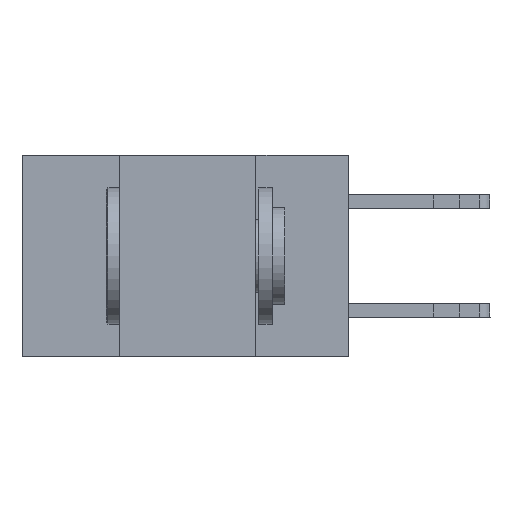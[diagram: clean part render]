
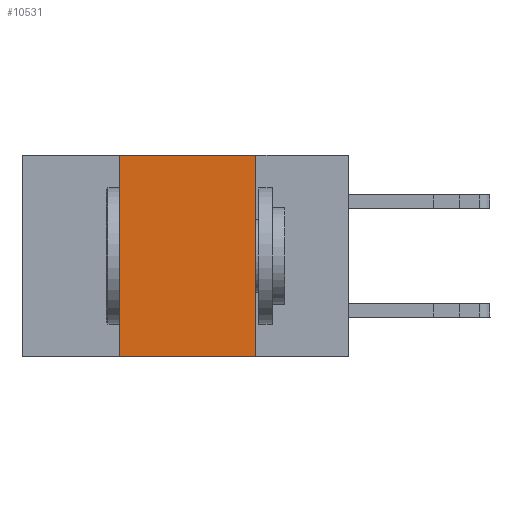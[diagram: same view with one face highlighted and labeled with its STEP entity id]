
A CAD part, left-side view. The second image highlights one B-rep face of the part: STEP entity #10531.
In plain terms, the highlighted planar face has unit normal (-1, 0, 0).
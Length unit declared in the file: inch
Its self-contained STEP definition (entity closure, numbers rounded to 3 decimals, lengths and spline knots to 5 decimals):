
#219 = DIRECTION ( 'NONE',  ( 0., 0., 1. ) ) ;
#605 = CARTESIAN_POINT ( 'NONE',  ( 0., 0.42, 0. ) ) ;
#889 = LINE ( 'NONE', #16623, #11078 ) ;
#1057 = DIRECTION ( 'NONE',  ( 1., 0., 0. ) ) ;
#1347 = DIRECTION ( 'NONE',  ( 0., 0., -1. ) ) ;
#1419 = EDGE_CURVE ( 'NONE', #9690, #16868, #15950, .T. ) ;
#1457 = CARTESIAN_POINT ( 'NONE',  ( 0., 0.6, 0. ) ) ;
#2435 = ORIENTED_EDGE ( 'NONE', *, *, #16948, .F. ) ;
#3744 = VECTOR ( 'NONE', #219, 39.37008 ) ;
#3847 = ORIENTED_EDGE ( 'NONE', *, *, #14532, .F. ) ;
#4110 = ORIENTED_EDGE ( 'NONE', *, *, #1419, .F. ) ;
#4305 = VECTOR ( 'NONE', #15871, 39.37008 ) ;
#4317 = PLANE ( 'NONE',  #13071 ) ;
#4586 = VECTOR ( 'NONE', #1347, 39.37008 ) ;
#4807 = CARTESIAN_POINT ( 'NONE',  ( 0., 0.6, 0. ) ) ;
#5170 = CARTESIAN_POINT ( 'NONE',  ( 0., 0.17, -0.37 ) ) ;
#5462 = EDGE_CURVE ( 'NONE', #10957, #16868, #889, .T. ) ;
#5676 = ORIENTED_EDGE ( 'NONE', *, *, #5462, .T. ) ;
#6406 = FACE_OUTER_BOUND ( 'NONE', #16677, .T. ) ;
#7031 = CARTESIAN_POINT ( 'NONE',  ( 0., 0.42, -0.37 ) ) ;
#7181 = LINE ( 'NONE', #1457, #4305 ) ;
#7282 = LINE ( 'NONE', #13332, #3744 ) ;
#7953 = CARTESIAN_POINT ( 'NONE',  ( 0., 0.17, 0. ) ) ;
#8764 = VERTEX_POINT ( 'NONE', #605 ) ;
#9690 = VERTEX_POINT ( 'NONE', #11444 ) ;
#10531 = ADVANCED_FACE ( 'NONE', ( #6406 ), #4317, .F. ) ;
#10957 = VERTEX_POINT ( 'NONE', #7031 ) ;
#11078 = VECTOR ( 'NONE', #13876, 39.37008 ) ;
#11444 = CARTESIAN_POINT ( 'NONE',  ( 0., 0.17, 0. ) ) ;
#13071 = AXIS2_PLACEMENT_3D ( 'NONE', #4807, #1057, #16893 ) ;
#13332 = CARTESIAN_POINT ( 'NONE',  ( 0., 0.42, 0. ) ) ;
#13876 = DIRECTION ( 'NONE',  ( 0., -1., 0. ) ) ;
#14532 = EDGE_CURVE ( 'NONE', #10957, #8764, #7282, .T. ) ;
#15871 = DIRECTION ( 'NONE',  ( 0., -1., 0. ) ) ;
#15950 = LINE ( 'NONE', #7953, #4586 ) ;
#16623 = CARTESIAN_POINT ( 'NONE',  ( 0., 0.6, -0.37 ) ) ;
#16677 = EDGE_LOOP ( 'NONE', ( #4110, #2435, #3847, #5676 ) ) ;
#16868 = VERTEX_POINT ( 'NONE', #5170 ) ;
#16893 = DIRECTION ( 'NONE',  ( 0., 0., -1. ) ) ;
#16948 = EDGE_CURVE ( 'NONE', #8764, #9690, #7181, .T. ) ;
